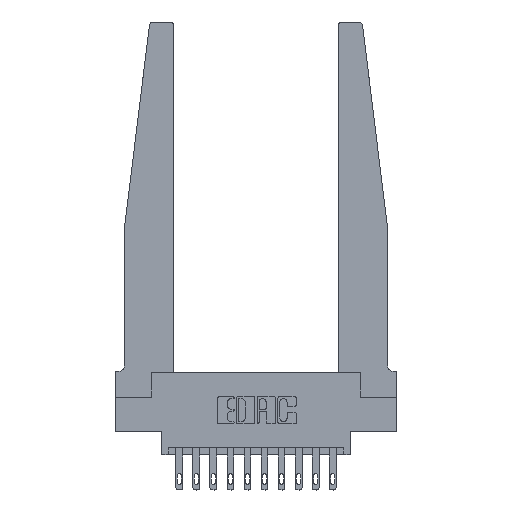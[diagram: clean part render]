
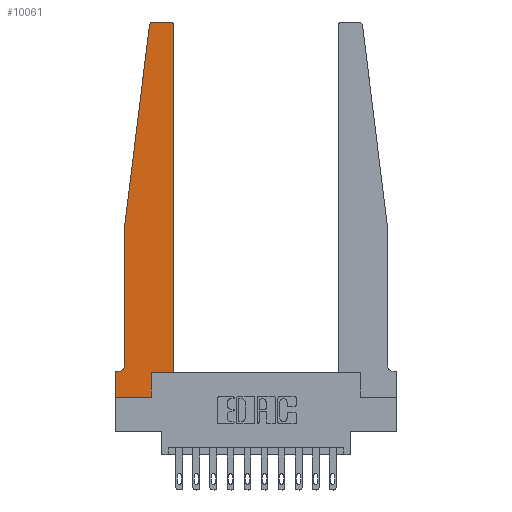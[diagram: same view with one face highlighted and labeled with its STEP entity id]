
A CAD part, top view. The second image highlights one B-rep face of the part: STEP entity #10061.
In plain terms, the highlighted planar face has unit normal (0, 0, 1).
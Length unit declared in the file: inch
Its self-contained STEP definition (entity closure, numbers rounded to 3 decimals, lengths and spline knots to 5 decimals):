
#137 = CARTESIAN_POINT ( 'NONE',  ( 0.27653, 2.75, 0.37 ) ) ;
#216 = EDGE_CURVE ( 'NONE', #514, #14012, #12822, .T. ) ;
#329 = AXIS2_PLACEMENT_3D ( 'NONE', #13143, #12987, #8092 ) ;
#349 = VERTEX_POINT ( 'NONE', #9696 ) ;
#514 = VERTEX_POINT ( 'NONE', #1695 ) ;
#1079 = VERTEX_POINT ( 'NONE', #137 ) ;
#1102 = LINE ( 'NONE', #10952, #7869 ) ;
#1125 = ORIENTED_EDGE ( 'NONE', *, *, #13657, .T. ) ;
#1230 = ORIENTED_EDGE ( 'NONE', *, *, #2988, .T. ) ;
#1552 = CIRCLE ( 'NONE', #4142, 0.03 ) ;
#1684 = VERTEX_POINT ( 'NONE', #1984 ) ;
#1695 = CARTESIAN_POINT ( 'NONE',  ( 0.015, 0.1875, 0.37 ) ) ;
#1831 = CARTESIAN_POINT ( 'NONE',  ( 0.425, 0.18, 0.37 ) ) ;
#1939 = VECTOR ( 'NONE', #12993, 39.37008 ) ;
#1977 = DIRECTION ( 'NONE',  ( 1., 0., 0. ) ) ;
#1984 = CARTESIAN_POINT ( 'NONE',  ( 0.425, 0.18, 0.37 ) ) ;
#2089 = CARTESIAN_POINT ( 'NONE',  ( 0.27653, 2.72, 0.37 ) ) ;
#2281 = CARTESIAN_POINT ( 'NONE',  ( 0.065, 0.2375, 0.37 ) ) ;
#2550 = CARTESIAN_POINT ( 'NONE',  ( 0.2605, 0., 0.37 ) ) ;
#2785 = DIRECTION ( 'NONE',  ( 0., -1., 0. ) ) ;
#2988 = EDGE_CURVE ( 'NONE', #15042, #514, #7333, .T. ) ;
#3308 = EDGE_CURVE ( 'NONE', #14012, #8535, #3775, .T. ) ;
#3665 = EDGE_CURVE ( 'NONE', #12742, #13686, #1102, .T. ) ;
#3775 = LINE ( 'NONE', #13943, #15158 ) ;
#3912 = AXIS2_PLACEMENT_3D ( 'NONE', #10194, #10033, #5127 ) ;
#4142 = AXIS2_PLACEMENT_3D ( 'NONE', #5464, #13202, #1977 ) ;
#4167 = CARTESIAN_POINT ( 'NONE',  ( 0., 0.1875, 0.37 ) ) ;
#4199 = CARTESIAN_POINT ( 'NONE',  ( 0., 0., 0.37 ) ) ;
#4255 = DIRECTION ( 'NONE',  ( -1., 0., 0. ) ) ;
#4323 = ORIENTED_EDGE ( 'NONE', *, *, #3665, .T. ) ;
#4432 = LINE ( 'NONE', #1831, #12006 ) ;
#4774 = CARTESIAN_POINT ( 'NONE',  ( 0.24675, 2.72367, 0.37 ) ) ;
#5127 = DIRECTION ( 'NONE',  ( 1., 0., 0. ) ) ;
#5178 = ORIENTED_EDGE ( 'NONE', *, *, #12078, .T. ) ;
#5207 = VECTOR ( 'NONE', #11563, 39.37008 ) ;
#5399 = AXIS2_PLACEMENT_3D ( 'NONE', #2089, #15995, #8427 ) ;
#5464 = CARTESIAN_POINT ( 'NONE',  ( 0.395, 2.72, 0.37 ) ) ;
#5479 = LINE ( 'NONE', #6796, #13338 ) ;
#5774 = ORIENTED_EDGE ( 'NONE', *, *, #8148, .T. ) ;
#5833 = CARTESIAN_POINT ( 'NONE',  ( 0.425, 2.72, 0.37 ) ) ;
#5855 = EDGE_LOOP ( 'NONE', ( #5774, #7063, #8591, #1125, #1230, #10421, #12977, #5178, #4323, #10995, #8160, #9856 ) ) ;
#6179 = CIRCLE ( 'NONE', #5399, 0.03 ) ;
#6247 = VECTOR ( 'NONE', #7172, 39.37008 ) ;
#6796 = CARTESIAN_POINT ( 'NONE',  ( 0.065, 1.25, 0.37 ) ) ;
#6806 = DIRECTION ( 'NONE',  ( 0., 1., 0. ) ) ;
#7063 = ORIENTED_EDGE ( 'NONE', *, *, #15894, .T. ) ;
#7172 = DIRECTION ( 'NONE',  ( -0.122, -0.992, 0. ) ) ;
#7249 = LINE ( 'NONE', #13608, #6247 ) ;
#7333 = CIRCLE ( 'NONE', #329, 0.05 ) ;
#7501 = PLANE ( 'NONE',  #3912 ) ;
#7753 = CARTESIAN_POINT ( 'NONE',  ( 0., 0., 0.37 ) ) ;
#7869 = VECTOR ( 'NONE', #11195, 39.37008 ) ;
#7996 = CARTESIAN_POINT ( 'NONE',  ( 0.065, 0.1875, 0.37 ) ) ;
#8092 = DIRECTION ( 'NONE',  ( -1., 0., 0. ) ) ;
#8148 = EDGE_CURVE ( 'NONE', #349, #1079, #13220, .T. ) ;
#8160 = ORIENTED_EDGE ( 'NONE', *, *, #9450, .T. ) ;
#8241 = CARTESIAN_POINT ( 'NONE',  ( 0.2605, 0.18, 0.37 ) ) ;
#8427 = DIRECTION ( 'NONE',  ( 1., 0., 0. ) ) ;
#8535 = VERTEX_POINT ( 'NONE', #7753 ) ;
#8591 = ORIENTED_EDGE ( 'NONE', *, *, #8816, .T. ) ;
#8726 = FACE_OUTER_BOUND ( 'NONE', #5855, .T. ) ;
#8816 = EDGE_CURVE ( 'NONE', #15450, #10459, #7249, .T. ) ;
#8967 = EDGE_CURVE ( 'NONE', #13686, #1684, #10415, .T. ) ;
#9421 = CARTESIAN_POINT ( 'NONE',  ( 0.065, 1.25, 0.37 ) ) ;
#9450 = EDGE_CURVE ( 'NONE', #1684, #13336, #4432, .T. ) ;
#9696 = CARTESIAN_POINT ( 'NONE',  ( 0.395, 2.75, 0.37 ) ) ;
#9856 = ORIENTED_EDGE ( 'NONE', *, *, #9861, .T. ) ;
#9861 = EDGE_CURVE ( 'NONE', #13336, #349, #1552, .T. ) ;
#10033 = DIRECTION ( 'NONE',  ( 0., 0., 1. ) ) ;
#10061 = ADVANCED_FACE ( 'NONE', ( #8726 ), #7501, .T. ) ;
#10194 = CARTESIAN_POINT ( 'NONE',  ( 0., 0.1875, 0.37 ) ) ;
#10310 = DIRECTION ( 'NONE',  ( 1., 0., 0. ) ) ;
#10415 = LINE ( 'NONE', #14086, #5207 ) ;
#10421 = ORIENTED_EDGE ( 'NONE', *, *, #216, .T. ) ;
#10454 = CARTESIAN_POINT ( 'NONE',  ( 0.25, 2.75, 0.37 ) ) ;
#10459 = VERTEX_POINT ( 'NONE', #9421 ) ;
#10465 = LINE ( 'NONE', #4199, #10474 ) ;
#10474 = VECTOR ( 'NONE', #10310, 39.37008 ) ;
#10952 = CARTESIAN_POINT ( 'NONE',  ( 0.2605, 0.18, 0.37 ) ) ;
#10995 = ORIENTED_EDGE ( 'NONE', *, *, #8967, .T. ) ;
#11195 = DIRECTION ( 'NONE',  ( 0., 1., 0. ) ) ;
#11563 = DIRECTION ( 'NONE',  ( 1., 0., 0. ) ) ;
#11756 = DIRECTION ( 'NONE',  ( 0., -1., 0. ) ) ;
#12006 = VECTOR ( 'NONE', #6806, 39.37008 ) ;
#12078 = EDGE_CURVE ( 'NONE', #8535, #12742, #10465, .T. ) ;
#12742 = VERTEX_POINT ( 'NONE', #2550 ) ;
#12822 = LINE ( 'NONE', #7996, #15366 ) ;
#12977 = ORIENTED_EDGE ( 'NONE', *, *, #3308, .T. ) ;
#12987 = DIRECTION ( 'NONE',  ( 0., 0., -1. ) ) ;
#12993 = DIRECTION ( 'NONE',  ( -1., 0., 0. ) ) ;
#13143 = CARTESIAN_POINT ( 'NONE',  ( 0.015, 0.2375, 0.37 ) ) ;
#13202 = DIRECTION ( 'NONE',  ( 0., 0., 1. ) ) ;
#13220 = LINE ( 'NONE', #10454, #1939 ) ;
#13336 = VERTEX_POINT ( 'NONE', #5833 ) ;
#13338 = VECTOR ( 'NONE', #11756, 39.37008 ) ;
#13608 = CARTESIAN_POINT ( 'NONE',  ( 0.065, 1.25, 0.37 ) ) ;
#13657 = EDGE_CURVE ( 'NONE', #10459, #15042, #5479, .T. ) ;
#13686 = VERTEX_POINT ( 'NONE', #8241 ) ;
#13943 = CARTESIAN_POINT ( 'NONE',  ( 0., 0., 0.37 ) ) ;
#14012 = VERTEX_POINT ( 'NONE', #4167 ) ;
#14086 = CARTESIAN_POINT ( 'NONE',  ( 0.425, 0.18, 0.37 ) ) ;
#15042 = VERTEX_POINT ( 'NONE', #2281 ) ;
#15158 = VECTOR ( 'NONE', #2785, 39.37008 ) ;
#15366 = VECTOR ( 'NONE', #4255, 39.37008 ) ;
#15450 = VERTEX_POINT ( 'NONE', #4774 ) ;
#15894 = EDGE_CURVE ( 'NONE', #1079, #15450, #6179, .T. ) ;
#15995 = DIRECTION ( 'NONE',  ( 0., 0., 1. ) ) ;
